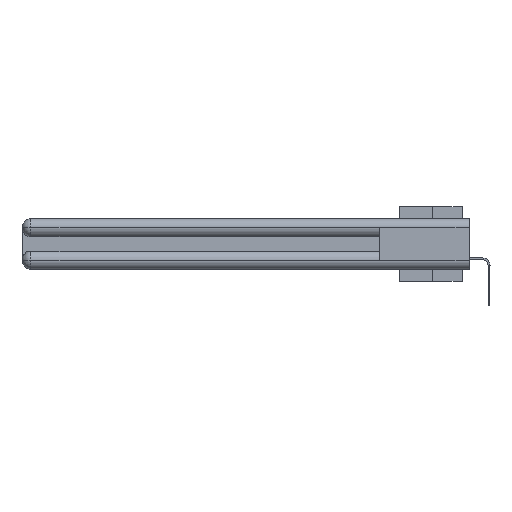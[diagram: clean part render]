
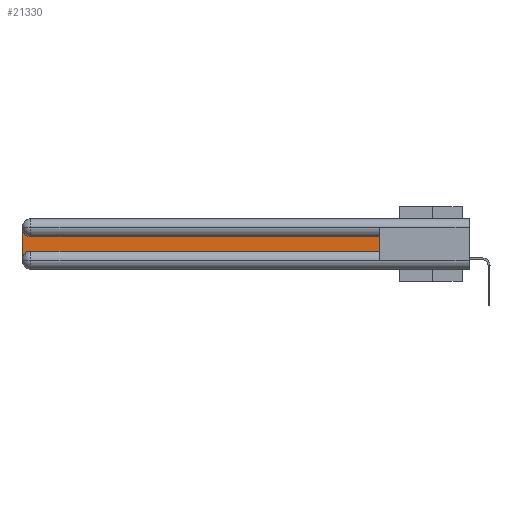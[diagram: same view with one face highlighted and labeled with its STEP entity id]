
A CAD part, left-side view. The second image highlights one B-rep face of the part: STEP entity #21330.
In plain terms, the highlighted planar face has unit normal (-1, 0, 0).
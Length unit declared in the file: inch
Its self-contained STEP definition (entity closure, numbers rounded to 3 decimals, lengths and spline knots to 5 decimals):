
#88 = VERTEX_POINT ( 'NONE', #19129 ) ;
#347 = CARTESIAN_POINT ( 'NONE',  ( 0.075, 3., -0.1225 ) ) ;
#1123 = DIRECTION ( 'NONE',  ( 0., 0., -1. ) ) ;
#3068 = EDGE_CURVE ( 'NONE', #88, #21103, #17926, .T. ) ;
#4412 = AXIS2_PLACEMENT_3D ( 'NONE', #347, #7008, #6911 ) ;
#5695 = VECTOR ( 'NONE', #22023, 39.37008 ) ;
#6070 = CARTESIAN_POINT ( 'NONE',  ( 0.075, 2.94, -0.1225 ) ) ;
#6496 = LINE ( 'NONE', #7894, #6837 ) ;
#6646 = EDGE_CURVE ( 'NONE', #21103, #11660, #8756, .T. ) ;
#6730 = CARTESIAN_POINT ( 'NONE',  ( 0.075, 3., -0.0625 ) ) ;
#6737 = PLANE ( 'NONE',  #4412 ) ;
#6837 = VECTOR ( 'NONE', #19282, 39.37008 ) ;
#6911 = DIRECTION ( 'NONE',  ( 0., 0., -1. ) ) ;
#7008 = DIRECTION ( 'NONE',  ( 1., 0., 0. ) ) ;
#7048 = EDGE_CURVE ( 'NONE', #19164, #17210, #21821, .T. ) ;
#7687 = DIRECTION ( 'NONE',  ( 1., 0., 0. ) ) ;
#7838 = ORIENTED_EDGE ( 'NONE', *, *, #19971, .T. ) ;
#7894 = CARTESIAN_POINT ( 'NONE',  ( 0.075, 0.6, -0.2175 ) ) ;
#8756 = LINE ( 'NONE', #27052, #5695 ) ;
#11408 = CIRCLE ( 'NONE', #14305, 0.06 ) ;
#11660 = VERTEX_POINT ( 'NONE', #24794 ) ;
#11923 = EDGE_CURVE ( 'NONE', #17210, #14921, #11408, .T. ) ;
#12855 = FACE_OUTER_BOUND ( 'NONE', #13772, .T. ) ;
#13252 = LINE ( 'NONE', #23902, #18859 ) ;
#13772 = EDGE_LOOP ( 'NONE', ( #26067, #14994, #7838, #27721, #22956, #15888 ) ) ;
#14305 = AXIS2_PLACEMENT_3D ( 'NONE', #17073, #19211, #21689 ) ;
#14921 = VERTEX_POINT ( 'NONE', #6730 ) ;
#14994 = ORIENTED_EDGE ( 'NONE', *, *, #11923, .T. ) ;
#15888 = ORIENTED_EDGE ( 'NONE', *, *, #18433, .T. ) ;
#16641 = CARTESIAN_POINT ( 'NONE',  ( 0.075, 2.94, -0.2175 ) ) ;
#17073 = CARTESIAN_POINT ( 'NONE',  ( 0.075, 2.94, -0.0625 ) ) ;
#17210 = VERTEX_POINT ( 'NONE', #6070 ) ;
#17354 = VECTOR ( 'NONE', #22108, 39.37008 ) ;
#17926 = CIRCLE ( 'NONE', #23377, 0.06 ) ;
#18433 = EDGE_CURVE ( 'NONE', #11660, #19164, #6496, .T. ) ;
#18859 = VECTOR ( 'NONE', #28361, 39.37008 ) ;
#19129 = CARTESIAN_POINT ( 'NONE',  ( 0.075, 3., -0.2775 ) ) ;
#19164 = VERTEX_POINT ( 'NONE', #23728 ) ;
#19211 = DIRECTION ( 'NONE',  ( 1., 0., 0. ) ) ;
#19282 = DIRECTION ( 'NONE',  ( 0., 0., 1. ) ) ;
#19971 = EDGE_CURVE ( 'NONE', #14921, #88, #13252, .T. ) ;
#20898 = CARTESIAN_POINT ( 'NONE',  ( 0.075, 2.94, -0.2775 ) ) ;
#21103 = VERTEX_POINT ( 'NONE', #16641 ) ;
#21330 = ADVANCED_FACE ( 'NONE', ( #12855 ), #6737, .F. ) ;
#21689 = DIRECTION ( 'NONE',  ( 0., 0., -1. ) ) ;
#21821 = LINE ( 'NONE', #22767, #17354 ) ;
#22023 = DIRECTION ( 'NONE',  ( 0., -1., 0. ) ) ;
#22108 = DIRECTION ( 'NONE',  ( 0., 1., 0. ) ) ;
#22767 = CARTESIAN_POINT ( 'NONE',  ( 0.075, 0.6, -0.1225 ) ) ;
#22956 = ORIENTED_EDGE ( 'NONE', *, *, #6646, .T. ) ;
#23377 = AXIS2_PLACEMENT_3D ( 'NONE', #20898, #7687, #1123 ) ;
#23728 = CARTESIAN_POINT ( 'NONE',  ( 0.075, 0.6, -0.1225 ) ) ;
#23902 = CARTESIAN_POINT ( 'NONE',  ( 0.075, 3., -0.2175 ) ) ;
#24794 = CARTESIAN_POINT ( 'NONE',  ( 0.075, 0.6, -0.2175 ) ) ;
#26067 = ORIENTED_EDGE ( 'NONE', *, *, #7048, .T. ) ;
#27052 = CARTESIAN_POINT ( 'NONE',  ( 0.075, 0.6, -0.2175 ) ) ;
#27721 = ORIENTED_EDGE ( 'NONE', *, *, #3068, .T. ) ;
#28361 = DIRECTION ( 'NONE',  ( 0., 0., -1. ) ) ;
